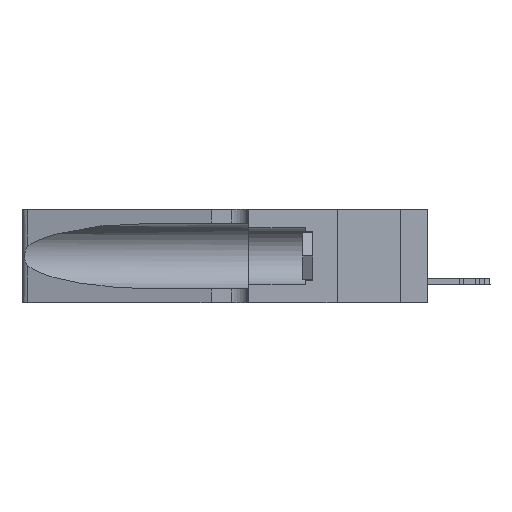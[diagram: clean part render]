
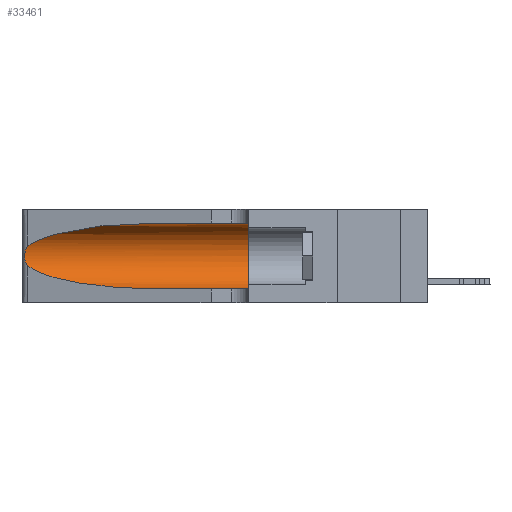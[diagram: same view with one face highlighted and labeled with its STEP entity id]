
A CAD part, left-side view. The second image highlights one B-rep face of the part: STEP entity #33461.
In plain terms, the highlighted cylindrical face has radius 3.308 mm (diameter 6.617 mm), a partial arc.
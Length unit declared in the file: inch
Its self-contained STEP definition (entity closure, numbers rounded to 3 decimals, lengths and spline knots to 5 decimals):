
#700 = VECTOR ( 'NONE', #26330, 39.37008 ) ;
#1088 = CARTESIAN_POINT ( 'NONE',  ( 0.1305, 0.72297, 0.05475 ) ) ;
#1103 =( BOUNDED_CURVE ( )  B_SPLINE_CURVE ( 3, ( #19955, #12928, #35005, #12775 ),
 .UNSPECIFIED., .F., .F. ) 
 B_SPLINE_CURVE_WITH_KNOTS ( ( 4, 4 ),
 ( 1.5708, 2.84003 ),
 .UNSPECIFIED. ) 
 CURVE ( )  GEOMETRIC_REPRESENTATION_ITEM ( )  RATIONAL_B_SPLINE_CURVE ( ( 1., 0.87, 0.87, 1. ) ) 
 REPRESENTATION_ITEM ( '' )  );
#1536 = CARTESIAN_POINT ( 'NONE',  ( 0.1305, 0.35, 0.185 ) ) ;
#1849 = CARTESIAN_POINT ( 'NONE',  ( 0.25487, 1.22718, 0.22369 ) ) ;
#2389 = CARTESIAN_POINT ( 'NONE',  ( 0.1305, 1.61858, 0.185 ) ) ;
#2906 = DIRECTION ( 'NONE',  ( 0., -1., 0. ) ) ;
#4059 = LINE ( 'NONE', #36404, #13974 ) ;
#4590 = CARTESIAN_POINT ( 'NONE',  ( 0.26075, 1.23896, 0.19203 ) ) ;
#6693 = VERTEX_POINT ( 'NONE', #23573 ) ;
#7317 = ORIENTED_EDGE ( 'NONE', *, *, #8919, .T. ) ;
#7545 = CARTESIAN_POINT ( 'NONE',  ( 0.18966, 0.96281, 0.05475 ) ) ;
#7568 = VERTEX_POINT ( 'NONE', #31823 ) ;
#7842 = CARTESIAN_POINT ( 'NONE',  ( 0.1305, 0.72297, 0.05475 ) ) ;
#7937 = VERTEX_POINT ( 'NONE', #1088 ) ;
#8526 = CARTESIAN_POINT ( 'NONE',  ( 0.26017, 1.23833, 0.17102 ) ) ;
#8919 = EDGE_CURVE ( 'NONE', #7568, #31437, #1103, .T. ) ;
#10716 = LINE ( 'NONE', #14919, #700 ) ;
#11876 = CARTESIAN_POINT ( 'NONE',  ( 0.25487, 1.22718, 0.14631 ) ) ;
#12391 = CARTESIAN_POINT ( 'NONE',  ( 0.25487, 1.22718, 0.22369 ) ) ;
#12775 = CARTESIAN_POINT ( 'NONE',  ( 0.25487, 1.22718, 0.22369 ) ) ;
#12816 = DIRECTION ( 'NONE',  ( 0., 1., 0. ) ) ;
#12928 = CARTESIAN_POINT ( 'NONE',  ( 0.18966, 0.96281, 0.31525 ) ) ;
#13974 = VECTOR ( 'NONE', #2906, 39.37008 ) ;
#14524 = VERTEX_POINT ( 'NONE', #36905 ) ;
#14919 = CARTESIAN_POINT ( 'NONE',  ( 0.1305, 1.61858, 0.31525 ) ) ;
#14959 = EDGE_CURVE ( 'NONE', #7937, #6693, #4059, .T. ) ;
#15961 = CARTESIAN_POINT ( 'NONE',  ( 0.26018, 1.23835, 0.19895 ) ) ;
#16138 = CARTESIAN_POINT ( 'NONE',  ( 0.25856, 1.23593, 0.16098 ) ) ;
#17230 = DIRECTION ( 'NONE',  ( 0., 0., -1. ) ) ;
#19398 = CARTESIAN_POINT ( 'NONE',  ( 0.25555, 1.22993, 0.14849 ) ) ;
#19557 = CARTESIAN_POINT ( 'NONE',  ( 0.25787, 1.23484, 0.2124 ) ) ;
#19728 = CARTESIAN_POINT ( 'NONE',  ( 0.26075, 1.23896, 0.178 ) ) ;
#19955 = CARTESIAN_POINT ( 'NONE',  ( 0.1305, 0.72297, 0.31525 ) ) ;
#20236 = AXIS2_PLACEMENT_3D ( 'NONE', #2389, #28492, #17230 ) ;
#20467 = ORIENTED_EDGE ( 'NONE', *, *, #14959, .T. ) ;
#20893 = EDGE_CURVE ( 'NONE', #14524, #6693, #26903, .T. ) ;
#23210 = CARTESIAN_POINT ( 'NONE',  ( 0.25639, 1.23186, 0.15144 ) ) ;
#23573 = CARTESIAN_POINT ( 'NONE',  ( 0.1305, 0.35, 0.05475 ) ) ;
#26330 = DIRECTION ( 'NONE',  ( 0., -1., 0. ) ) ;
#26568 = AXIS2_PLACEMENT_3D ( 'NONE', #1536, #12816, #31881 ) ;
#26903 = CIRCLE ( 'NONE', #26568, 0.13025 ) ;
#28492 = DIRECTION ( 'NONE',  ( 0., -1., 0. ) ) ;
#28804 = B_SPLINE_CURVE_WITH_KNOTS ( 'NONE', 3,
 ( #12391, #34931, #38588, #19557, #38761, #15961, #4590, #19728, #8526, #16138, #46251, #23210, #19398, #42499 ),
 .UNSPECIFIED., .F., .F.,
 ( 4, 2, 2, 2, 2, 2, 4 ),
 ( 0., 0.00027, 0.00053, 0.00107, 0.0016, 0.00187, 0.00214 ),
 .UNSPECIFIED. ) ;
#30319 = CARTESIAN_POINT ( 'NONE',  ( 0.2373, 1.15595, 0.08982 ) ) ;
#31437 = VERTEX_POINT ( 'NONE', #1849 ) ;
#31823 = CARTESIAN_POINT ( 'NONE',  ( 0.1305, 0.72297, 0.31525 ) ) ;
#31881 = DIRECTION ( 'NONE',  ( 0., 0., 1. ) ) ;
#32439 = CARTESIAN_POINT ( 'NONE',  ( 0.25487, 1.22718, 0.14631 ) ) ;
#32834 = ORIENTED_EDGE ( 'NONE', *, *, #40893, .F. ) ;
#33461 = ADVANCED_FACE ( 'NONE', ( #37187 ), #38335, .F. ) ;
#34075 = ORIENTED_EDGE ( 'NONE', *, *, #44947, .T. ) ;
#34623 = ORIENTED_EDGE ( 'NONE', *, *, #39146, .T. ) ;
#34931 = CARTESIAN_POINT ( 'NONE',  ( 0.25555, 1.22994, 0.2215 ) ) ;
#35005 = CARTESIAN_POINT ( 'NONE',  ( 0.2373, 1.15595, 0.28018 ) ) ;
#36404 = CARTESIAN_POINT ( 'NONE',  ( 0.1305, 1.61858, 0.05475 ) ) ;
#36905 = CARTESIAN_POINT ( 'NONE',  ( 0.1305, 0.35, 0.31525 ) ) ;
#37187 = FACE_OUTER_BOUND ( 'NONE', #39108, .T. ) ;
#38335 = CYLINDRICAL_SURFACE ( 'NONE', #20236, 0.13025 ) ;
#38588 = CARTESIAN_POINT ( 'NONE',  ( 0.25639, 1.23184, 0.21858 ) ) ;
#38761 = CARTESIAN_POINT ( 'NONE',  ( 0.25854, 1.2359, 0.20912 ) ) ;
#39108 = EDGE_LOOP ( 'NONE', ( #7317, #34623, #34075, #20467, #40263, #32834 ) ) ;
#39146 = EDGE_CURVE ( 'NONE', #31437, #39457, #28804, .T. ) ;
#39457 = VERTEX_POINT ( 'NONE', #32439 ) ;
#40263 = ORIENTED_EDGE ( 'NONE', *, *, #20893, .F. ) ;
#40893 = EDGE_CURVE ( 'NONE', #7568, #14524, #10716, .T. ) ;
#42499 = CARTESIAN_POINT ( 'NONE',  ( 0.25487, 1.22718, 0.14631 ) ) ;
#44802 =( BOUNDED_CURVE ( )  B_SPLINE_CURVE ( 3, ( #11876, #30319, #7545, #7842 ),
 .UNSPECIFIED., .F., .F. ) 
 B_SPLINE_CURVE_WITH_KNOTS ( ( 4, 4 ),
 ( 3.44316, 4.71239 ),
 .UNSPECIFIED. ) 
 CURVE ( )  GEOMETRIC_REPRESENTATION_ITEM ( )  RATIONAL_B_SPLINE_CURVE ( ( 1., 0.87, 0.87, 1. ) ) 
 REPRESENTATION_ITEM ( '' )  );
#44947 = EDGE_CURVE ( 'NONE', #39457, #7937, #44802, .T. ) ;
#46251 = CARTESIAN_POINT ( 'NONE',  ( 0.25789, 1.23486, 0.15765 ) ) ;
